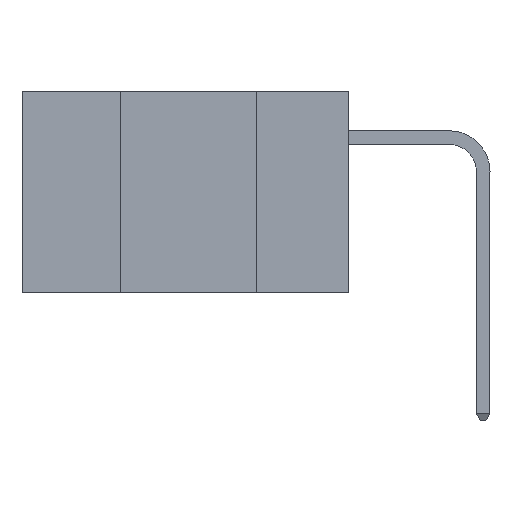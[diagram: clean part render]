
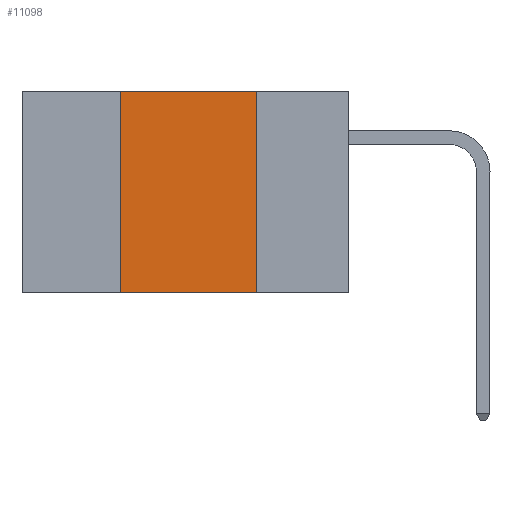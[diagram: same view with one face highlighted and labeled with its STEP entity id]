
A CAD part, left-side view. The second image highlights one B-rep face of the part: STEP entity #11098.
In plain terms, the highlighted planar face has unit normal (-1, 0, 0).
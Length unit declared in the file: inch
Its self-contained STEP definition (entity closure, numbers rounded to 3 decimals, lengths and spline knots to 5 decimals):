
#613 = CARTESIAN_POINT ( 'NONE',  ( 0., 0.6, -0.37 ) ) ;
#1178 = DIRECTION ( 'NONE',  ( 1., 0., 0. ) ) ;
#2249 = VERTEX_POINT ( 'NONE', #21068 ) ;
#2311 = VERTEX_POINT ( 'NONE', #9539 ) ;
#2954 = VECTOR ( 'NONE', #4024, 39.37008 ) ;
#3239 = EDGE_CURVE ( 'NONE', #6189, #2311, #3883, .T. ) ;
#3554 = LINE ( 'NONE', #18550, #20808 ) ;
#3584 = FACE_OUTER_BOUND ( 'NONE', #8958, .T. ) ;
#3883 = LINE ( 'NONE', #15717, #20309 ) ;
#3908 = EDGE_CURVE ( 'NONE', #2311, #19431, #3554, .T. ) ;
#4024 = DIRECTION ( 'NONE',  ( 0., -1., 0. ) ) ;
#6189 = VERTEX_POINT ( 'NONE', #13982 ) ;
#6548 = LINE ( 'NONE', #18127, #15023 ) ;
#7980 = DIRECTION ( 'NONE',  ( 0., 0., -1. ) ) ;
#8304 = DIRECTION ( 'NONE',  ( 0., 0., 1. ) ) ;
#8958 = EDGE_LOOP ( 'NONE', ( #12101, #12824, #13082, #17425 ) ) ;
#9539 = CARTESIAN_POINT ( 'NONE',  ( 0., 0.17, 0. ) ) ;
#11083 = CARTESIAN_POINT ( 'NONE',  ( 0., 0.6, 0. ) ) ;
#11098 = ADVANCED_FACE ( 'NONE', ( #3584 ), #14250, .F. ) ;
#11314 = DIRECTION ( 'NONE',  ( 0., -1., 0. ) ) ;
#11547 = AXIS2_PLACEMENT_3D ( 'NONE', #11083, #1178, #7980 ) ;
#12101 = ORIENTED_EDGE ( 'NONE', *, *, #3908, .F. ) ;
#12824 = ORIENTED_EDGE ( 'NONE', *, *, #3239, .F. ) ;
#13082 = ORIENTED_EDGE ( 'NONE', *, *, #14611, .F. ) ;
#13176 = CARTESIAN_POINT ( 'NONE',  ( 0., 0.17, -0.37 ) ) ;
#13982 = CARTESIAN_POINT ( 'NONE',  ( 0., 0.42, 0. ) ) ;
#14148 = EDGE_CURVE ( 'NONE', #2249, #19431, #17884, .T. ) ;
#14250 = PLANE ( 'NONE',  #11547 ) ;
#14611 = EDGE_CURVE ( 'NONE', #2249, #6189, #6548, .T. ) ;
#15023 = VECTOR ( 'NONE', #8304, 39.37008 ) ;
#15717 = CARTESIAN_POINT ( 'NONE',  ( 0., 0.6, 0. ) ) ;
#17425 = ORIENTED_EDGE ( 'NONE', *, *, #14148, .T. ) ;
#17884 = LINE ( 'NONE', #613, #2954 ) ;
#18127 = CARTESIAN_POINT ( 'NONE',  ( 0., 0.42, 0. ) ) ;
#18550 = CARTESIAN_POINT ( 'NONE',  ( 0., 0.17, 0. ) ) ;
#19431 = VERTEX_POINT ( 'NONE', #13176 ) ;
#20240 = DIRECTION ( 'NONE',  ( 0., 0., -1. ) ) ;
#20309 = VECTOR ( 'NONE', #11314, 39.37008 ) ;
#20808 = VECTOR ( 'NONE', #20240, 39.37008 ) ;
#21068 = CARTESIAN_POINT ( 'NONE',  ( 0., 0.42, -0.37 ) ) ;
